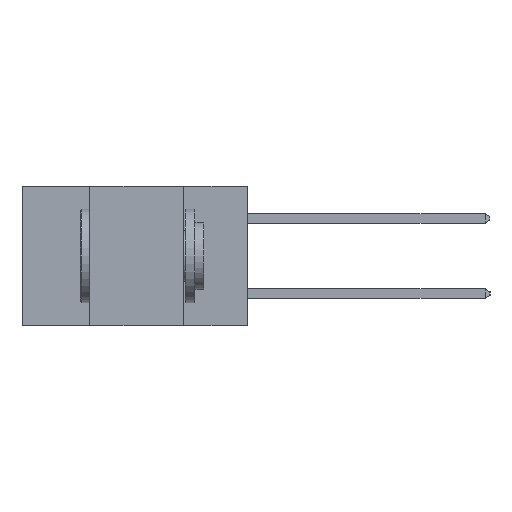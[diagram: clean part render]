
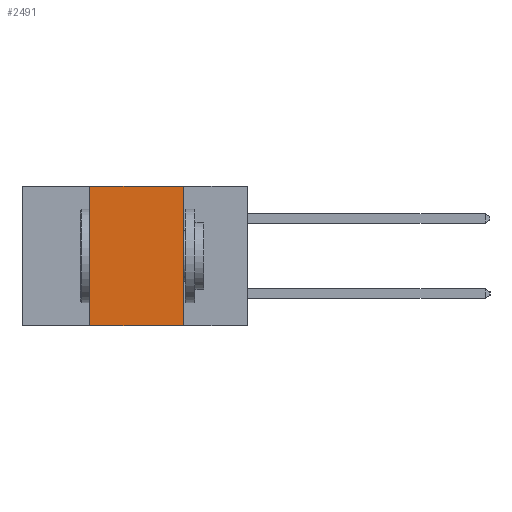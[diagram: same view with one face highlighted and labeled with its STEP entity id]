
A CAD part, left-side view. The second image highlights one B-rep face of the part: STEP entity #2491.
In plain terms, the highlighted planar face has unit normal (-1, 0, 0).
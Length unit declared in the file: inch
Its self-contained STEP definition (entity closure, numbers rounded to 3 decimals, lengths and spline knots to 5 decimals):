
#1039 = VECTOR ( 'NONE', #10290, 39.37008 ) ;
#1192 = VECTOR ( 'NONE', #9290, 39.37008 ) ;
#1359 = LINE ( 'NONE', #10206, #3494 ) ;
#1633 = CARTESIAN_POINT ( 'NONE',  ( 0., 0.6, 0. ) ) ;
#1730 = VERTEX_POINT ( 'NONE', #12350 ) ;
#2317 = PLANE ( 'NONE',  #3333 ) ;
#2351 = ORIENTED_EDGE ( 'NONE', *, *, #6133, .F. ) ;
#2459 = FACE_OUTER_BOUND ( 'NONE', #10204, .T. ) ;
#2491 = ADVANCED_FACE ( 'NONE', ( #2459 ), #2317, .F. ) ;
#3201 = ORIENTED_EDGE ( 'NONE', *, *, #6136, .F. ) ;
#3333 = AXIS2_PLACEMENT_3D ( 'NONE', #1633, #5403, #7339 ) ;
#3464 = ORIENTED_EDGE ( 'NONE', *, *, #6254, .F. ) ;
#3494 = VECTOR ( 'NONE', #10154, 39.37008 ) ;
#3599 = ORIENTED_EDGE ( 'NONE', *, *, #6302, .T. ) ;
#3957 = LINE ( 'NONE', #9364, #1192 ) ;
#4575 = LINE ( 'NONE', #9547, #9520 ) ;
#5397 = CARTESIAN_POINT ( 'NONE',  ( 0., 0.17, 0. ) ) ;
#5403 = DIRECTION ( 'NONE',  ( 1., 0., 0. ) ) ;
#6133 = EDGE_CURVE ( 'NONE', #6894, #1730, #9048, .T. ) ;
#6136 = EDGE_CURVE ( 'NONE', #10607, #6894, #1359, .T. ) ;
#6254 = EDGE_CURVE ( 'NONE', #11704, #10607, #4575, .T. ) ;
#6302 = EDGE_CURVE ( 'NONE', #11704, #1730, #3957, .T. ) ;
#6894 = VERTEX_POINT ( 'NONE', #5397 ) ;
#7339 = DIRECTION ( 'NONE',  ( 0., 0., -1. ) ) ;
#8437 = CARTESIAN_POINT ( 'NONE',  ( 0., 0.42, 0. ) ) ;
#9048 = LINE ( 'NONE', #10305, #1039 ) ;
#9290 = DIRECTION ( 'NONE',  ( 0., -1., 0. ) ) ;
#9364 = CARTESIAN_POINT ( 'NONE',  ( 0., 0.6, -0.37 ) ) ;
#9508 = DIRECTION ( 'NONE',  ( 0., 0., 1. ) ) ;
#9520 = VECTOR ( 'NONE', #9508, 39.37008 ) ;
#9547 = CARTESIAN_POINT ( 'NONE',  ( 0., 0.42, -0.37 ) ) ;
#10154 = DIRECTION ( 'NONE',  ( 0., -1., 0. ) ) ;
#10204 = EDGE_LOOP ( 'NONE', ( #2351, #3201, #3464, #3599 ) ) ;
#10206 = CARTESIAN_POINT ( 'NONE',  ( 0., 0.6, 0. ) ) ;
#10290 = DIRECTION ( 'NONE',  ( 0., 0., -1. ) ) ;
#10305 = CARTESIAN_POINT ( 'NONE',  ( 0., 0.17, -0.37 ) ) ;
#10607 = VERTEX_POINT ( 'NONE', #8437 ) ;
#10815 = CARTESIAN_POINT ( 'NONE',  ( 0., 0.42, -0.37 ) ) ;
#11704 = VERTEX_POINT ( 'NONE', #10815 ) ;
#12350 = CARTESIAN_POINT ( 'NONE',  ( 0., 0.17, -0.37 ) ) ;
